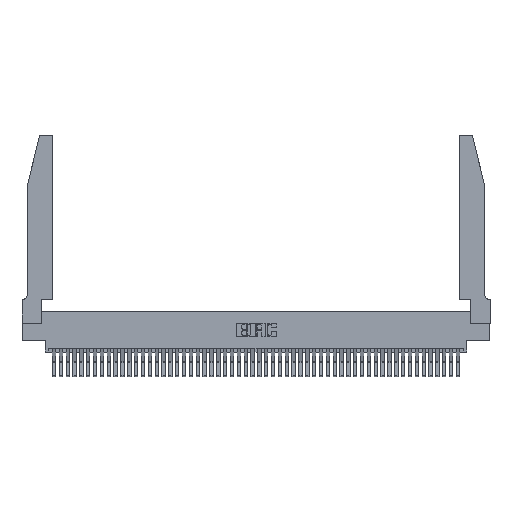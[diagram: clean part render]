
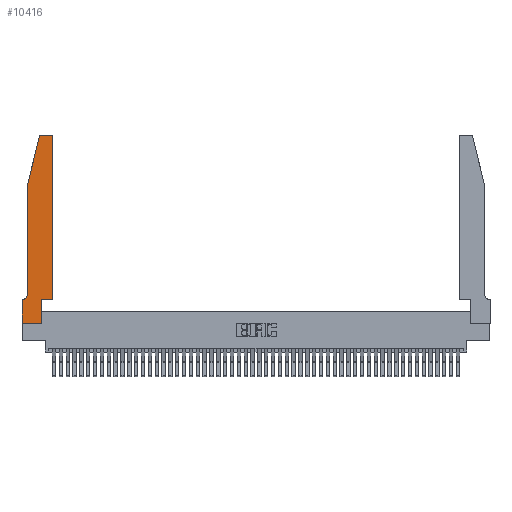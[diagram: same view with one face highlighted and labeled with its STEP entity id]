
A CAD part, top view. The second image highlights one B-rep face of the part: STEP entity #10416.
In plain terms, the highlighted planar face has unit normal (0, 0, 1).
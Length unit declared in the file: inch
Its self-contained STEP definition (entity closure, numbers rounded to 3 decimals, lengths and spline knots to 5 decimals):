
#614 = EDGE_CURVE ( 'NONE', #8526, #39900, #47352, .T. ) ;
#1486 = DIRECTION ( 'NONE',  ( 1., 0., 0. ) ) ;
#3310 = EDGE_CURVE ( 'NONE', #38982, #8526, #42440, .T. ) ;
#3664 = VERTEX_POINT ( 'NONE', #25698 ) ;
#4119 = ORIENTED_EDGE ( 'NONE', *, *, #42677, .T. ) ;
#6237 = CARTESIAN_POINT ( 'NONE',  ( 0.0755, 0.42, 0.37 ) ) ;
#6945 = VERTEX_POINT ( 'NONE', #49657 ) ;
#7569 = EDGE_CURVE ( 'NONE', #42315, #43889, #46207, .T. ) ;
#7710 = DIRECTION ( 'NONE',  ( 0., 1., 0. ) ) ;
#8526 = VERTEX_POINT ( 'NONE', #6237 ) ;
#9679 = ORIENTED_EDGE ( 'NONE', *, *, #3310, .T. ) ;
#9832 = CARTESIAN_POINT ( 'NONE',  ( 0.4505, 2.72, 0.37 ) ) ;
#9850 = CARTESIAN_POINT ( 'NONE',  ( 0.4205, 2.75, 0.37 ) ) ;
#10416 = ADVANCED_FACE ( 'NONE', ( #47378 ), #10832, .T. ) ;
#10832 = PLANE ( 'NONE',  #13661 ) ;
#10921 = ORIENTED_EDGE ( 'NONE', *, *, #614, .T. ) ;
#11361 = LINE ( 'NONE', #20651, #49435 ) ;
#12322 = CARTESIAN_POINT ( 'NONE',  ( 0., 0., 0.37 ) ) ;
#12737 = CARTESIAN_POINT ( 'NONE',  ( 0.25487, 2.72718, 0.37 ) ) ;
#13040 = DIRECTION ( 'NONE',  ( 0., -1., 0. ) ) ;
#13661 = AXIS2_PLACEMENT_3D ( 'NONE', #37567, #14893, #41547 ) ;
#13743 = CARTESIAN_POINT ( 'NONE',  ( 0.4505, 0.35, 0.37 ) ) ;
#13953 = VERTEX_POINT ( 'NONE', #9832 ) ;
#13976 = CARTESIAN_POINT ( 'NONE',  ( 0.2865, 0.35, 0.37 ) ) ;
#14046 = VECTOR ( 'NONE', #7710, 39.37008 ) ;
#14328 = VECTOR ( 'NONE', #43300, 39.37008 ) ;
#14780 = ORIENTED_EDGE ( 'NONE', *, *, #37515, .T. ) ;
#14893 = DIRECTION ( 'NONE',  ( 0., 0., 1. ) ) ;
#15648 = ORIENTED_EDGE ( 'NONE', *, *, #29452, .T. ) ;
#15920 = VECTOR ( 'NONE', #42824, 39.37008 ) ;
#16650 = VECTOR ( 'NONE', #48678, 39.37008 ) ;
#16971 = EDGE_CURVE ( 'NONE', #13953, #46194, #25841, .T. ) ;
#17197 = ORIENTED_EDGE ( 'NONE', *, *, #48058, .T. ) ;
#17691 = VERTEX_POINT ( 'NONE', #12737 ) ;
#17810 = CIRCLE ( 'NONE', #25249, 0.03 ) ;
#18445 = LINE ( 'NONE', #20726, #37507 ) ;
#18578 = DIRECTION ( 'NONE',  ( 0., 0., -1. ) ) ;
#19339 = EDGE_CURVE ( 'NONE', #46194, #6945, #18445, .T. ) ;
#20568 = DIRECTION ( 'NONE',  ( 0., 0., 1. ) ) ;
#20597 = CARTESIAN_POINT ( 'NONE',  ( 0.0755, 0.35, 0.37 ) ) ;
#20651 = CARTESIAN_POINT ( 'NONE',  ( 0., 0., 0.37 ) ) ;
#20726 = CARTESIAN_POINT ( 'NONE',  ( 0.2605, 2.75, 0.37 ) ) ;
#20789 = LINE ( 'NONE', #41281, #29691 ) ;
#20817 = LINE ( 'NONE', #13743, #48650 ) ;
#20819 = CARTESIAN_POINT ( 'NONE',  ( 0.0055, 0.35, 0.37 ) ) ;
#22228 = VECTOR ( 'NONE', #30357, 39.37008 ) ;
#23749 = CARTESIAN_POINT ( 'NONE',  ( 0., 0., 0.37 ) ) ;
#24731 = DIRECTION ( 'NONE',  ( 0., 0., 1. ) ) ;
#25249 = AXIS2_PLACEMENT_3D ( 'NONE', #47413, #24731, #1486 ) ;
#25608 = CARTESIAN_POINT ( 'NONE',  ( 0., 0.35, 0.37 ) ) ;
#25698 = CARTESIAN_POINT ( 'NONE',  ( 0.4505, 0.35, 0.37 ) ) ;
#25708 = LINE ( 'NONE', #20597, #14328 ) ;
#25841 = CIRCLE ( 'NONE', #38190, 0.03 ) ;
#26518 = CARTESIAN_POINT ( 'NONE',  ( 0.0755, 2., 0.37 ) ) ;
#26871 = EDGE_LOOP ( 'NONE', ( #29409, #49159, #15648, #9679, #10921, #4119, #36458, #38930, #34096, #17197, #14780, #37538 ) ) ;
#27991 = EDGE_CURVE ( 'NONE', #41983, #42315, #11361, .T. ) ;
#29409 = ORIENTED_EDGE ( 'NONE', *, *, #19339, .T. ) ;
#29452 = EDGE_CURVE ( 'NONE', #17691, #38982, #36910, .T. ) ;
#29691 = VECTOR ( 'NONE', #29826, 39.37008 ) ;
#29826 = DIRECTION ( 'NONE',  ( 0., 1., 0. ) ) ;
#29832 = CARTESIAN_POINT ( 'NONE',  ( 0.0755, 2., 0.37 ) ) ;
#30357 = DIRECTION ( 'NONE',  ( 0., -1., 0. ) ) ;
#34096 = ORIENTED_EDGE ( 'NONE', *, *, #38331, .T. ) ;
#34559 = CARTESIAN_POINT ( 'NONE',  ( 0.2865, 0.35, 0.37 ) ) ;
#35195 = AXIS2_PLACEMENT_3D ( 'NONE', #41367, #18578, #45120 ) ;
#36458 = ORIENTED_EDGE ( 'NONE', *, *, #27991, .T. ) ;
#36910 = LINE ( 'NONE', #29832, #16650 ) ;
#37507 = VECTOR ( 'NONE', #43430, 39.37008 ) ;
#37515 = EDGE_CURVE ( 'NONE', #3664, #13953, #20789, .T. ) ;
#37538 = ORIENTED_EDGE ( 'NONE', *, *, #16971, .T. ) ;
#37567 = CARTESIAN_POINT ( 'NONE',  ( 0., 0.35, 0.37 ) ) ;
#38190 = AXIS2_PLACEMENT_3D ( 'NONE', #43275, #20568, #47057 ) ;
#38331 = EDGE_CURVE ( 'NONE', #43889, #47386, #44421, .T. ) ;
#38930 = ORIENTED_EDGE ( 'NONE', *, *, #7569, .T. ) ;
#38982 = VERTEX_POINT ( 'NONE', #42146 ) ;
#39900 = VERTEX_POINT ( 'NONE', #20819 ) ;
#41281 = CARTESIAN_POINT ( 'NONE',  ( 0.4505, 0.35, 0.37 ) ) ;
#41367 = CARTESIAN_POINT ( 'NONE',  ( 0.0055, 0.42, 0.37 ) ) ;
#41547 = DIRECTION ( 'NONE',  ( 1., 0., 0. ) ) ;
#41983 = VERTEX_POINT ( 'NONE', #25608 ) ;
#42146 = CARTESIAN_POINT ( 'NONE',  ( 0.0755, 2., 0.37 ) ) ;
#42315 = VERTEX_POINT ( 'NONE', #23749 ) ;
#42440 = LINE ( 'NONE', #26518, #22228 ) ;
#42677 = EDGE_CURVE ( 'NONE', #39900, #41983, #25708, .T. ) ;
#42824 = DIRECTION ( 'NONE',  ( 1., 0., 0. ) ) ;
#43275 = CARTESIAN_POINT ( 'NONE',  ( 0.4205, 2.72, 0.37 ) ) ;
#43300 = DIRECTION ( 'NONE',  ( -1., 0., 0. ) ) ;
#43430 = DIRECTION ( 'NONE',  ( -1., 0., 0. ) ) ;
#43889 = VERTEX_POINT ( 'NONE', #47151 ) ;
#44203 = DIRECTION ( 'NONE',  ( 1., 0., 0. ) ) ;
#44421 = LINE ( 'NONE', #34559, #14046 ) ;
#44610 = EDGE_CURVE ( 'NONE', #6945, #17691, #17810, .T. ) ;
#45120 = DIRECTION ( 'NONE',  ( -1., 0., 0. ) ) ;
#46194 = VERTEX_POINT ( 'NONE', #9850 ) ;
#46207 = LINE ( 'NONE', #12322, #15920 ) ;
#47057 = DIRECTION ( 'NONE',  ( 1., 0., 0. ) ) ;
#47151 = CARTESIAN_POINT ( 'NONE',  ( 0.2865, 0., 0.37 ) ) ;
#47352 = CIRCLE ( 'NONE', #35195, 0.07 ) ;
#47378 = FACE_OUTER_BOUND ( 'NONE', #26871, .T. ) ;
#47386 = VERTEX_POINT ( 'NONE', #13976 ) ;
#47413 = CARTESIAN_POINT ( 'NONE',  ( 0.284, 2.72, 0.37 ) ) ;
#48058 = EDGE_CURVE ( 'NONE', #47386, #3664, #20817, .T. ) ;
#48650 = VECTOR ( 'NONE', #44203, 39.37008 ) ;
#48678 = DIRECTION ( 'NONE',  ( -0.239, -0.971, 0. ) ) ;
#49159 = ORIENTED_EDGE ( 'NONE', *, *, #44610, .T. ) ;
#49435 = VECTOR ( 'NONE', #13040, 39.37008 ) ;
#49657 = CARTESIAN_POINT ( 'NONE',  ( 0.284, 2.75, 0.37 ) ) ;
